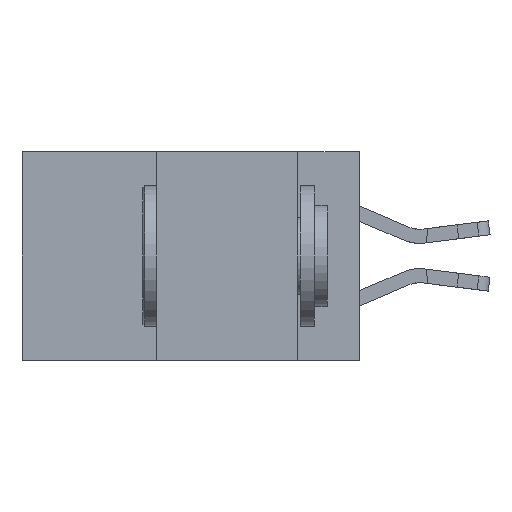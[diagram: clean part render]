
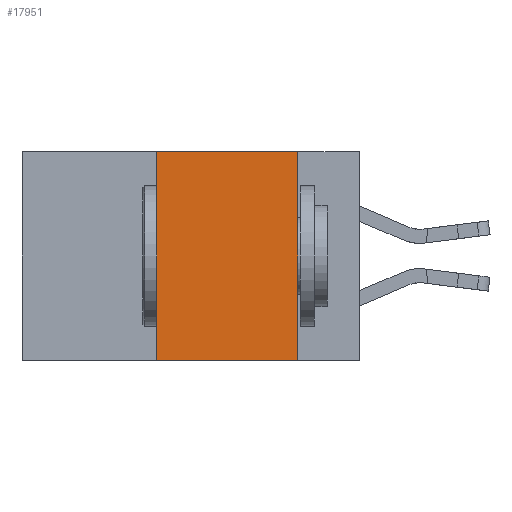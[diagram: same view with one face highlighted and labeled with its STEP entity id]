
A CAD part, left-side view. The second image highlights one B-rep face of the part: STEP entity #17951.
In plain terms, the highlighted planar face has unit normal (-1, 0, 0).
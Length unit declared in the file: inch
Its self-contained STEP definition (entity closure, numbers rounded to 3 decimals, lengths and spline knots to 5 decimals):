
#1105 = DIRECTION ( 'NONE',  ( 0., -1., 0. ) ) ;
#2319 = CARTESIAN_POINT ( 'NONE',  ( 0., 0.36, -0.37 ) ) ;
#2736 = CARTESIAN_POINT ( 'NONE',  ( 0., 0.36, 0. ) ) ;
#2886 = VERTEX_POINT ( 'NONE', #15622 ) ;
#3430 = VECTOR ( 'NONE', #18265, 39.37008 ) ;
#4806 = VERTEX_POINT ( 'NONE', #22711 ) ;
#4904 = EDGE_CURVE ( 'NONE', #4806, #14813, #18311, .T. ) ;
#5217 = EDGE_CURVE ( 'NONE', #14813, #2886, #25861, .T. ) ;
#7324 = PLANE ( 'NONE',  #15684 ) ;
#8678 = CARTESIAN_POINT ( 'NONE',  ( 0., 0.6, -0.37 ) ) ;
#10233 = EDGE_CURVE ( 'NONE', #26880, #4806, #19899, .T. ) ;
#11689 = CARTESIAN_POINT ( 'NONE',  ( 0., 0.6, 0. ) ) ;
#11776 = DIRECTION ( 'NONE',  ( 0., 0., -1. ) ) ;
#12720 = CARTESIAN_POINT ( 'NONE',  ( 0., 0.11, 0. ) ) ;
#12842 = DIRECTION ( 'NONE',  ( 0., -1., 0. ) ) ;
#13194 = CARTESIAN_POINT ( 'NONE',  ( 0., 0.6, 0. ) ) ;
#14813 = VERTEX_POINT ( 'NONE', #12720 ) ;
#15622 = CARTESIAN_POINT ( 'NONE',  ( 0., 0.11, -0.37 ) ) ;
#15684 = AXIS2_PLACEMENT_3D ( 'NONE', #11689, #18433, #11776 ) ;
#16041 = ORIENTED_EDGE ( 'NONE', *, *, #10233, .F. ) ;
#16312 = ORIENTED_EDGE ( 'NONE', *, *, #4904, .F. ) ;
#16536 = ORIENTED_EDGE ( 'NONE', *, *, #5217, .F. ) ;
#17499 = EDGE_CURVE ( 'NONE', #26880, #2886, #27398, .T. ) ;
#17951 = ADVANCED_FACE ( 'NONE', ( #24639 ), #7324, .F. ) ;
#18265 = DIRECTION ( 'NONE',  ( 0., 0., 1. ) ) ;
#18269 = ORIENTED_EDGE ( 'NONE', *, *, #17499, .T. ) ;
#18311 = LINE ( 'NONE', #13194, #23409 ) ;
#18433 = DIRECTION ( 'NONE',  ( 1., 0., 0. ) ) ;
#19899 = LINE ( 'NONE', #2736, #3430 ) ;
#20144 = VECTOR ( 'NONE', #12842, 39.37008 ) ;
#21280 = EDGE_LOOP ( 'NONE', ( #16536, #16312, #16041, #18269 ) ) ;
#21546 = CARTESIAN_POINT ( 'NONE',  ( 0., 0.11, 0. ) ) ;
#22711 = CARTESIAN_POINT ( 'NONE',  ( 0., 0.36, 0. ) ) ;
#23409 = VECTOR ( 'NONE', #1105, 39.37008 ) ;
#24639 = FACE_OUTER_BOUND ( 'NONE', #21280, .T. ) ;
#25861 = LINE ( 'NONE', #21546, #28250 ) ;
#26880 = VERTEX_POINT ( 'NONE', #2319 ) ;
#27398 = LINE ( 'NONE', #8678, #20144 ) ;
#27478 = DIRECTION ( 'NONE',  ( 0., 0., -1. ) ) ;
#28250 = VECTOR ( 'NONE', #27478, 39.37008 ) ;
